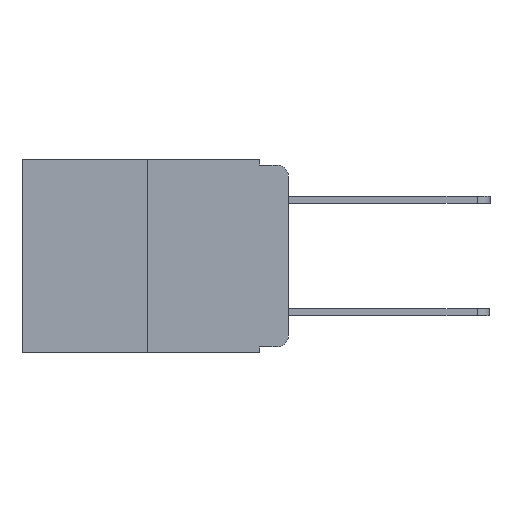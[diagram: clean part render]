
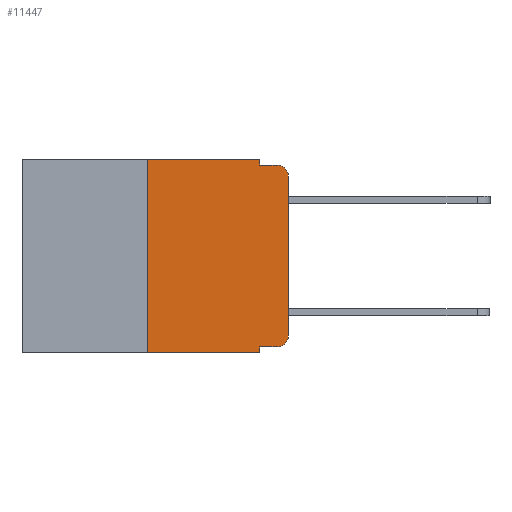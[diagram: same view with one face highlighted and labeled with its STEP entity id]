
A CAD part, left-side view. The second image highlights one B-rep face of the part: STEP entity #11447.
In plain terms, the highlighted planar face has unit normal (-1, 0, 0).
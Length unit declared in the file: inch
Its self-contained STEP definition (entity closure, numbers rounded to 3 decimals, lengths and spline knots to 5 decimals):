
#325 = DIRECTION ( 'NONE',  ( 0., -1., 0. ) ) ;
#386 = ORIENTED_EDGE ( 'NONE', *, *, #10986, .T. ) ;
#875 = CARTESIAN_POINT ( 'NONE',  ( 0., 0.25, 0. ) ) ;
#1349 = DIRECTION ( 'NONE',  ( -1., 0., 0. ) ) ;
#1512 = CARTESIAN_POINT ( 'NONE',  ( 0., 0., 0. ) ) ;
#1522 = CARTESIAN_POINT ( 'NONE',  ( 0., 0.02, -0.01 ) ) ;
#1586 = DIRECTION ( 'NONE',  ( 0., 0., 1. ) ) ;
#1797 = VERTEX_POINT ( 'NONE', #14851 ) ;
#1989 = CARTESIAN_POINT ( 'NONE',  ( 0., 0.051, -0.333 ) ) ;
#2054 = DIRECTION ( 'NONE',  ( -1., 0., 0. ) ) ;
#2241 = VECTOR ( 'NONE', #325, 39.37008 ) ;
#2543 = VECTOR ( 'NONE', #6976, 39.37008 ) ;
#2689 = CARTESIAN_POINT ( 'NONE',  ( 0., 0.473, 0. ) ) ;
#2746 = EDGE_LOOP ( 'NONE', ( #14078, #16330, #17772, #18170, #12110, #10367, #14611, #8330, #386, #10152 ) ) ;
#2955 = LINE ( 'NONE', #875, #18138 ) ;
#3310 = EDGE_CURVE ( 'NONE', #14964, #15509, #12623, .T. ) ;
#3418 = AXIS2_PLACEMENT_3D ( 'NONE', #2689, #13377, #4387 ) ;
#3736 = VECTOR ( 'NONE', #1586, 39.37008 ) ;
#4106 = AXIS2_PLACEMENT_3D ( 'NONE', #11342, #2054, #12778 ) ;
#4243 = DIRECTION ( 'NONE',  ( 0., -1., 0. ) ) ;
#4382 = LINE ( 'NONE', #11786, #8123 ) ;
#4387 = DIRECTION ( 'NONE',  ( 0., 0., -1. ) ) ;
#4672 = VECTOR ( 'NONE', #7977, 39.37008 ) ;
#4695 = VECTOR ( 'NONE', #17071, 39.37008 ) ;
#6167 = FACE_OUTER_BOUND ( 'NONE', #2746, .T. ) ;
#6185 = LINE ( 'NONE', #12763, #2241 ) ;
#6893 = CIRCLE ( 'NONE', #18819, 0.02 ) ;
#6976 = DIRECTION ( 'NONE',  ( 0., 0., -1. ) ) ;
#7445 = DIRECTION ( 'NONE',  ( 0., 0., 1. ) ) ;
#7553 = VERTEX_POINT ( 'NONE', #13371 ) ;
#7716 = CARTESIAN_POINT ( 'NONE',  ( 0., 0.051, -0.01 ) ) ;
#7977 = DIRECTION ( 'NONE',  ( 0., -1., 0. ) ) ;
#8123 = VECTOR ( 'NONE', #4243, 39.37008 ) ;
#8330 = ORIENTED_EDGE ( 'NONE', *, *, #17960, .F. ) ;
#9311 = EDGE_CURVE ( 'NONE', #13467, #14964, #17795, .T. ) ;
#9320 = VERTEX_POINT ( 'NONE', #9976 ) ;
#9327 = LINE ( 'NONE', #15752, #4695 ) ;
#9913 = CARTESIAN_POINT ( 'NONE',  ( 0., 0.051, 0. ) ) ;
#9976 = CARTESIAN_POINT ( 'NONE',  ( 0., 0., -0.03 ) ) ;
#10068 = CARTESIAN_POINT ( 'NONE',  ( 0., 0.25, -0.343 ) ) ;
#10152 = ORIENTED_EDGE ( 'NONE', *, *, #10663, .T. ) ;
#10367 = ORIENTED_EDGE ( 'NONE', *, *, #19182, .F. ) ;
#10663 = EDGE_CURVE ( 'NONE', #7553, #13108, #6893, .T. ) ;
#10791 = CARTESIAN_POINT ( 'NONE',  ( 0., 0.02, -0.313 ) ) ;
#10986 = EDGE_CURVE ( 'NONE', #12922, #7553, #6185, .T. ) ;
#11236 = LINE ( 'NONE', #12315, #18183 ) ;
#11275 = VERTEX_POINT ( 'NONE', #14446 ) ;
#11342 = CARTESIAN_POINT ( 'NONE',  ( 0., 0.02, -0.03 ) ) ;
#11447 = ADVANCED_FACE ( 'NONE', ( #6167 ), #16141, .F. ) ;
#11722 = CIRCLE ( 'NONE', #4106, 0.02 ) ;
#11786 = CARTESIAN_POINT ( 'NONE',  ( 0., 0.473, 0. ) ) ;
#11841 = LINE ( 'NONE', #1512, #3736 ) ;
#12110 = ORIENTED_EDGE ( 'NONE', *, *, #17702, .F. ) ;
#12199 = DIRECTION ( 'NONE',  ( 0., 0., -1. ) ) ;
#12315 = CARTESIAN_POINT ( 'NONE',  ( 0., 0.051, 0. ) ) ;
#12623 = LINE ( 'NONE', #13662, #4672 ) ;
#12763 = CARTESIAN_POINT ( 'NONE',  ( 0., 0.051, -0.333 ) ) ;
#12778 = DIRECTION ( 'NONE',  ( 0., 0., -1. ) ) ;
#12922 = VERTEX_POINT ( 'NONE', #1989 ) ;
#13108 = VERTEX_POINT ( 'NONE', #18684 ) ;
#13371 = CARTESIAN_POINT ( 'NONE',  ( 0., 0.02, -0.333 ) ) ;
#13377 = DIRECTION ( 'NONE',  ( 1., 0., 0. ) ) ;
#13394 = VERTEX_POINT ( 'NONE', #10068 ) ;
#13467 = VERTEX_POINT ( 'NONE', #17282 ) ;
#13662 = CARTESIAN_POINT ( 'NONE',  ( 0., 0.051, -0.01 ) ) ;
#13809 = DIRECTION ( 'NONE',  ( 0., 0., -1. ) ) ;
#14078 = ORIENTED_EDGE ( 'NONE', *, *, #15164, .T. ) ;
#14446 = CARTESIAN_POINT ( 'NONE',  ( 0., 0.051, -0.343 ) ) ;
#14611 = ORIENTED_EDGE ( 'NONE', *, *, #17034, .T. ) ;
#14851 = CARTESIAN_POINT ( 'NONE',  ( 0., 0.25, 0. ) ) ;
#14964 = VERTEX_POINT ( 'NONE', #7716 ) ;
#15164 = EDGE_CURVE ( 'NONE', #13108, #9320, #11841, .T. ) ;
#15509 = VERTEX_POINT ( 'NONE', #1522 ) ;
#15752 = CARTESIAN_POINT ( 'NONE',  ( 0., 0.473, -0.343 ) ) ;
#16141 = PLANE ( 'NONE',  #3418 ) ;
#16330 = ORIENTED_EDGE ( 'NONE', *, *, #17524, .T. ) ;
#17034 = EDGE_CURVE ( 'NONE', #13394, #11275, #9327, .T. ) ;
#17071 = DIRECTION ( 'NONE',  ( 0., -1., 0. ) ) ;
#17282 = CARTESIAN_POINT ( 'NONE',  ( 0., 0.051, 0. ) ) ;
#17524 = EDGE_CURVE ( 'NONE', #9320, #15509, #11722, .T. ) ;
#17702 = EDGE_CURVE ( 'NONE', #1797, #13467, #4382, .T. ) ;
#17772 = ORIENTED_EDGE ( 'NONE', *, *, #3310, .F. ) ;
#17795 = LINE ( 'NONE', #9913, #2543 ) ;
#17960 = EDGE_CURVE ( 'NONE', #12922, #11275, #11236, .T. ) ;
#18138 = VECTOR ( 'NONE', #7445, 39.37008 ) ;
#18170 = ORIENTED_EDGE ( 'NONE', *, *, #9311, .F. ) ;
#18183 = VECTOR ( 'NONE', #13809, 39.37008 ) ;
#18684 = CARTESIAN_POINT ( 'NONE',  ( 0., 0., -0.313 ) ) ;
#18819 = AXIS2_PLACEMENT_3D ( 'NONE', #10791, #1349, #12199 ) ;
#19182 = EDGE_CURVE ( 'NONE', #13394, #1797, #2955, .T. ) ;
